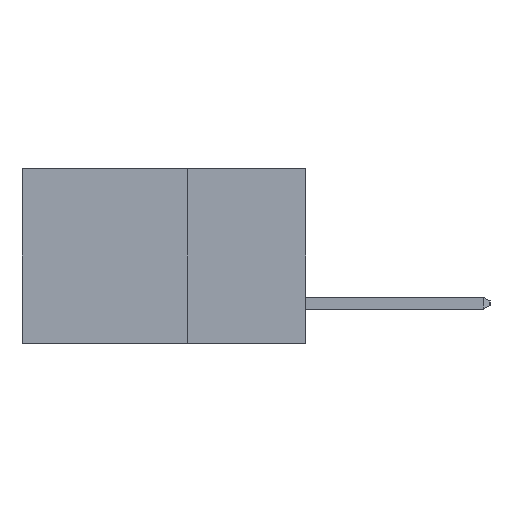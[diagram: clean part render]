
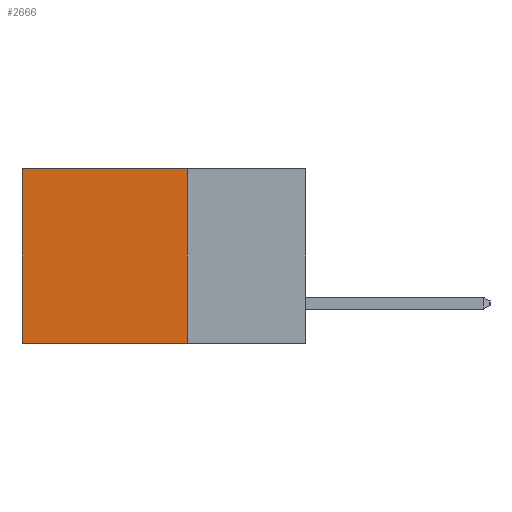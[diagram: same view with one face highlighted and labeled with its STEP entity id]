
A CAD part, left-side view. The second image highlights one B-rep face of the part: STEP entity #2666.
In plain terms, the highlighted planar face has unit normal (-1, 0, 0).
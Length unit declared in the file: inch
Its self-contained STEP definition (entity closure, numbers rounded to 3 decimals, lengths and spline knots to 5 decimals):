
#259 = EDGE_CURVE ( 'NONE', #11760, #343, #3441, .T. ) ;
#343 = VERTEX_POINT ( 'NONE', #14296 ) ;
#745 = EDGE_CURVE ( 'NONE', #11760, #9976, #3570, .T. ) ;
#1361 = ORIENTED_EDGE ( 'NONE', *, *, #14527, .T. ) ;
#1678 = DIRECTION ( 'NONE',  ( 0., 1., 0. ) ) ;
#1728 = CARTESIAN_POINT ( 'NONE',  ( 0.298, 0.25, 0. ) ) ;
#2666 = ADVANCED_FACE ( 'NONE', ( #14848 ), #10778, .F. ) ;
#3441 = LINE ( 'NONE', #9346, #13080 ) ;
#3523 = CARTESIAN_POINT ( 'NONE',  ( 0.298, 0.25, -0.37 ) ) ;
#3570 = LINE ( 'NONE', #13060, #16720 ) ;
#4310 = ORIENTED_EDGE ( 'NONE', *, *, #6983, .F. ) ;
#4714 = CARTESIAN_POINT ( 'NONE',  ( 0.298, 0.25, -0.37 ) ) ;
#6903 = DIRECTION ( 'NONE',  ( 0., 1., 0. ) ) ;
#6983 = EDGE_CURVE ( 'NONE', #9976, #13248, #14125, .T. ) ;
#8437 = CARTESIAN_POINT ( 'NONE',  ( 0.298, 0.6, 0. ) ) ;
#8649 = EDGE_LOOP ( 'NONE', ( #1361, #4310, #17045, #11907 ) ) ;
#9140 = LINE ( 'NONE', #8437, #12199 ) ;
#9346 = CARTESIAN_POINT ( 'NONE',  ( 0.298, 0.25, 0. ) ) ;
#9358 = CARTESIAN_POINT ( 'NONE',  ( 0.298, 0.25, 0. ) ) ;
#9976 = VERTEX_POINT ( 'NONE', #3523 ) ;
#10659 = VECTOR ( 'NONE', #1678, 39.37008 ) ;
#10778 = PLANE ( 'NONE',  #15836 ) ;
#11760 = VERTEX_POINT ( 'NONE', #9358 ) ;
#11907 = ORIENTED_EDGE ( 'NONE', *, *, #259, .T. ) ;
#12199 = VECTOR ( 'NONE', #16314, 39.37008 ) ;
#12364 = DIRECTION ( 'NONE',  ( 0., 0., -1. ) ) ;
#13060 = CARTESIAN_POINT ( 'NONE',  ( 0.298, 0.25, 0. ) ) ;
#13080 = VECTOR ( 'NONE', #6903, 39.37008 ) ;
#13162 = DIRECTION ( 'NONE',  ( 0., 0., -1. ) ) ;
#13248 = VERTEX_POINT ( 'NONE', #16583 ) ;
#14125 = LINE ( 'NONE', #4714, #10659 ) ;
#14296 = CARTESIAN_POINT ( 'NONE',  ( 0.298, 0.6, 0. ) ) ;
#14527 = EDGE_CURVE ( 'NONE', #343, #13248, #9140, .T. ) ;
#14848 = FACE_OUTER_BOUND ( 'NONE', #8649, .T. ) ;
#15570 = DIRECTION ( 'NONE',  ( 1., 0., 0. ) ) ;
#15836 = AXIS2_PLACEMENT_3D ( 'NONE', #1728, #15570, #13162 ) ;
#16314 = DIRECTION ( 'NONE',  ( 0., 0., -1. ) ) ;
#16583 = CARTESIAN_POINT ( 'NONE',  ( 0.298, 0.6, -0.37 ) ) ;
#16720 = VECTOR ( 'NONE', #12364, 39.37008 ) ;
#17045 = ORIENTED_EDGE ( 'NONE', *, *, #745, .F. ) ;
